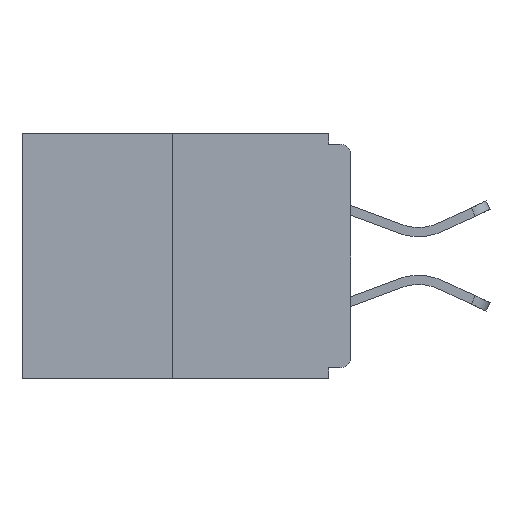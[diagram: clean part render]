
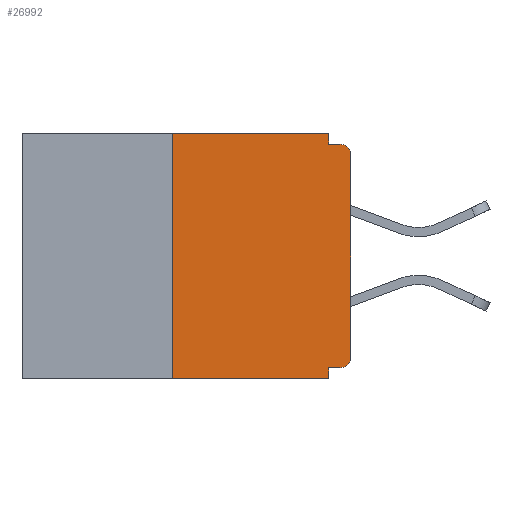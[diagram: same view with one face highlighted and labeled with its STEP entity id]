
A CAD part, left-side view. The second image highlights one B-rep face of the part: STEP entity #26992.
In plain terms, the highlighted planar face has unit normal (-1, 0, 0).
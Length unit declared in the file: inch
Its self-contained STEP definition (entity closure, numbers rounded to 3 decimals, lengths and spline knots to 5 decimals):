
#24 = LINE ( 'NONE', #23802, #8288 ) ;
#36 = ORIENTED_EDGE ( 'NONE', *, *, #1905, .F. ) ;
#89 = CIRCLE ( 'NONE', #11473, 0.015 ) ;
#137 = CARTESIAN_POINT ( 'NONE',  ( 0., 0.015, -0.03 ) ) ;
#283 = CARTESIAN_POINT ( 'NONE',  ( 0., 0., 0. ) ) ;
#312 = ORIENTED_EDGE ( 'NONE', *, *, #18143, .F. ) ;
#397 = VERTEX_POINT ( 'NONE', #22190 ) ;
#409 = DIRECTION ( 'NONE',  ( 0., 0., -1. ) ) ;
#1163 = ORIENTED_EDGE ( 'NONE', *, *, #1677, .T. ) ;
#1507 = AXIS2_PLACEMENT_3D ( 'NONE', #27445, #10294, #12505 ) ;
#1677 = EDGE_CURVE ( 'NONE', #5603, #21317, #9310, .T. ) ;
#1905 = EDGE_CURVE ( 'NONE', #9623, #14137, #3061, .T. ) ;
#2596 = VERTEX_POINT ( 'NONE', #19081 ) ;
#2782 = ORIENTED_EDGE ( 'NONE', *, *, #26003, .F. ) ;
#3033 = ORIENTED_EDGE ( 'NONE', *, *, #16893, .T. ) ;
#3061 = LINE ( 'NONE', #7367, #16591 ) ;
#3692 = VECTOR ( 'NONE', #16920, 39.37008 ) ;
#3916 = FACE_OUTER_BOUND ( 'NONE', #25431, .T. ) ;
#4083 = DIRECTION ( 'NONE',  ( 0., 0., -1. ) ) ;
#4968 = CARTESIAN_POINT ( 'NONE',  ( 0., 0.031, 0. ) ) ;
#5408 = ORIENTED_EDGE ( 'NONE', *, *, #8504, .T. ) ;
#5452 = CARTESIAN_POINT ( 'NONE',  ( 0., 0.25, 0. ) ) ;
#5603 = VERTEX_POINT ( 'NONE', #16535 ) ;
#6129 = CARTESIAN_POINT ( 'NONE',  ( 0., 0.46, 0. ) ) ;
#6472 = CIRCLE ( 'NONE', #1507, 0.015 ) ;
#7367 = CARTESIAN_POINT ( 'NONE',  ( 0., 0.46, 0. ) ) ;
#7474 = DIRECTION ( 'NONE',  ( 0., 0., 1. ) ) ;
#7754 = VERTEX_POINT ( 'NONE', #26253 ) ;
#7935 = VECTOR ( 'NONE', #18424, 39.37008 ) ;
#8014 = LINE ( 'NONE', #12834, #14962 ) ;
#8288 = VECTOR ( 'NONE', #409, 39.37008 ) ;
#8504 = EDGE_CURVE ( 'NONE', #27293, #5603, #6472, .T. ) ;
#8727 = DIRECTION ( 'NONE',  ( 0., 0., -1. ) ) ;
#9310 = LINE ( 'NONE', #283, #3692 ) ;
#9623 = VERTEX_POINT ( 'NONE', #16403 ) ;
#9792 = EDGE_CURVE ( 'NONE', #21317, #12251, #89, .T. ) ;
#10294 = DIRECTION ( 'NONE',  ( -1., 0., 0. ) ) ;
#11222 = EDGE_CURVE ( 'NONE', #397, #12251, #22854, .T. ) ;
#11473 = AXIS2_PLACEMENT_3D ( 'NONE', #137, #21357, #8727 ) ;
#12208 = CARTESIAN_POINT ( 'NONE',  ( 0., 0.031, -0.343 ) ) ;
#12251 = VERTEX_POINT ( 'NONE', #22869 ) ;
#12257 = LINE ( 'NONE', #18114, #21932 ) ;
#12505 = DIRECTION ( 'NONE',  ( 0., 0., -1. ) ) ;
#12581 = DIRECTION ( 'NONE',  ( 1., 0., 0. ) ) ;
#12741 = AXIS2_PLACEMENT_3D ( 'NONE', #6129, #12581, #4083 ) ;
#12834 = CARTESIAN_POINT ( 'NONE',  ( 0., 0.46, -0.343 ) ) ;
#13760 = DIRECTION ( 'NONE',  ( 0., -1., 0. ) ) ;
#13977 = CARTESIAN_POINT ( 'NONE',  ( 0., 0.031, 0. ) ) ;
#14137 = VERTEX_POINT ( 'NONE', #4968 ) ;
#14962 = VECTOR ( 'NONE', #18772, 39.37008 ) ;
#15244 = ORIENTED_EDGE ( 'NONE', *, *, #9792, .T. ) ;
#16403 = CARTESIAN_POINT ( 'NONE',  ( 0., 0.25, 0. ) ) ;
#16535 = CARTESIAN_POINT ( 'NONE',  ( 0., 0., -0.313 ) ) ;
#16591 = VECTOR ( 'NONE', #13760, 39.37008 ) ;
#16633 = DIRECTION ( 'NONE',  ( 0., 1., 0. ) ) ;
#16893 = EDGE_CURVE ( 'NONE', #7754, #17970, #8014, .T. ) ;
#16920 = DIRECTION ( 'NONE',  ( 0., 0., 1. ) ) ;
#17657 = EDGE_CURVE ( 'NONE', #27293, #2596, #12257, .T. ) ;
#17951 = ORIENTED_EDGE ( 'NONE', *, *, #22799, .F. ) ;
#17970 = VERTEX_POINT ( 'NONE', #12208 ) ;
#18114 = CARTESIAN_POINT ( 'NONE',  ( 0., 0., -0.328 ) ) ;
#18143 = EDGE_CURVE ( 'NONE', #2596, #17970, #24, .T. ) ;
#18424 = DIRECTION ( 'NONE',  ( 0., 0., -1. ) ) ;
#18670 = CARTESIAN_POINT ( 'NONE',  ( 0., 0.015, -0.328 ) ) ;
#18772 = DIRECTION ( 'NONE',  ( 0., -1., 0. ) ) ;
#18858 = CARTESIAN_POINT ( 'NONE',  ( 0., 0., -0.03 ) ) ;
#19081 = CARTESIAN_POINT ( 'NONE',  ( 0., 0.031, -0.328 ) ) ;
#19237 = LINE ( 'NONE', #13977, #7935 ) ;
#19809 = ORIENTED_EDGE ( 'NONE', *, *, #11222, .F. ) ;
#20762 = LINE ( 'NONE', #5452, #24372 ) ;
#20815 = ORIENTED_EDGE ( 'NONE', *, *, #17657, .F. ) ;
#21317 = VERTEX_POINT ( 'NONE', #18858 ) ;
#21357 = DIRECTION ( 'NONE',  ( -1., 0., 0. ) ) ;
#21546 = VECTOR ( 'NONE', #21963, 39.37008 ) ;
#21932 = VECTOR ( 'NONE', #16633, 39.37008 ) ;
#21963 = DIRECTION ( 'NONE',  ( 0., -1., 0. ) ) ;
#22190 = CARTESIAN_POINT ( 'NONE',  ( 0., 0.031, -0.015 ) ) ;
#22799 = EDGE_CURVE ( 'NONE', #7754, #9623, #20762, .T. ) ;
#22854 = LINE ( 'NONE', #24245, #21546 ) ;
#22869 = CARTESIAN_POINT ( 'NONE',  ( 0., 0.015, -0.015 ) ) ;
#23165 = PLANE ( 'NONE',  #12741 ) ;
#23802 = CARTESIAN_POINT ( 'NONE',  ( 0., 0.031, -0.343 ) ) ;
#24245 = CARTESIAN_POINT ( 'NONE',  ( 0., 0., -0.015 ) ) ;
#24372 = VECTOR ( 'NONE', #7474, 39.37008 ) ;
#25431 = EDGE_LOOP ( 'NONE', ( #36, #17951, #3033, #312, #20815, #5408, #1163, #15244, #19809, #2782 ) ) ;
#26003 = EDGE_CURVE ( 'NONE', #14137, #397, #19237, .T. ) ;
#26253 = CARTESIAN_POINT ( 'NONE',  ( 0., 0.25, -0.343 ) ) ;
#26992 = ADVANCED_FACE ( 'NONE', ( #3916 ), #23165, .F. ) ;
#27293 = VERTEX_POINT ( 'NONE', #18670 ) ;
#27445 = CARTESIAN_POINT ( 'NONE',  ( 0., 0.015, -0.313 ) ) ;
